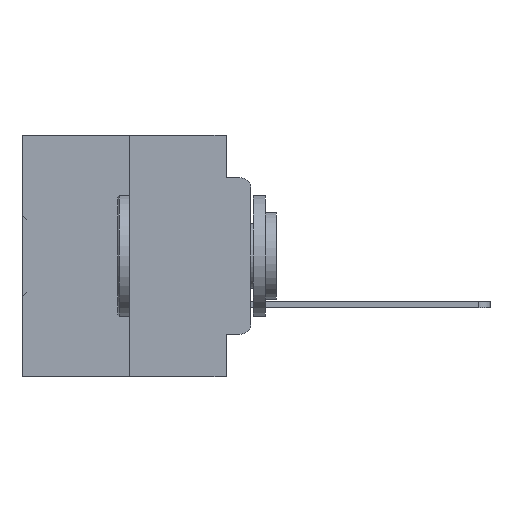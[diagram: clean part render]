
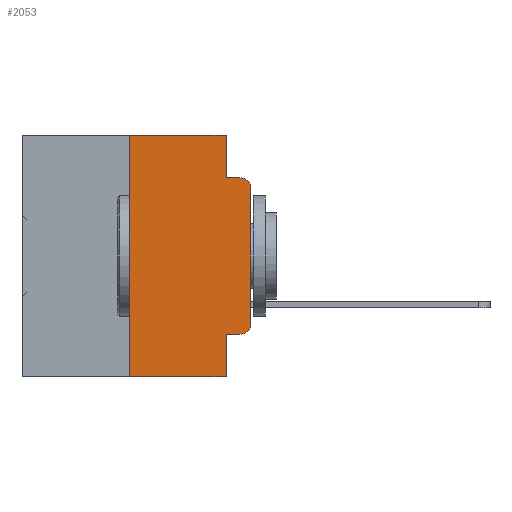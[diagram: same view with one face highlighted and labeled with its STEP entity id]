
A CAD part, left-side view. The second image highlights one B-rep face of the part: STEP entity #2053.
In plain terms, the highlighted planar face has unit normal (-1, 0, 0).
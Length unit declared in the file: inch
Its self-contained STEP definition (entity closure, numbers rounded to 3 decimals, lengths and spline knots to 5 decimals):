
#136 = EDGE_CURVE ( 'NONE', #15803, #18637, #18666, .T. ) ;
#483 = VECTOR ( 'NONE', #5728, 39.37008 ) ;
#659 = CARTESIAN_POINT ( 'NONE',  ( 0., 0.051, 0. ) ) ;
#1601 = VECTOR ( 'NONE', #25866, 39.37008 ) ;
#1630 = DIRECTION ( 'NONE',  ( 0., 0., -1. ) ) ;
#2053 = ADVANCED_FACE ( 'NONE', ( #24489 ), #9906, .F. ) ;
#2297 = ORIENTED_EDGE ( 'NONE', *, *, #10276, .F. ) ;
#2713 = CARTESIAN_POINT ( 'NONE',  ( 0., 0., 0. ) ) ;
#2790 = CARTESIAN_POINT ( 'NONE',  ( 0., 0., -0.1085 ) ) ;
#3482 = EDGE_CURVE ( 'NONE', #35715, #7925, #32908, .T. ) ;
#3700 = VERTEX_POINT ( 'NONE', #659 ) ;
#3823 = ORIENTED_EDGE ( 'NONE', *, *, #28074, .T. ) ;
#4172 = VERTEX_POINT ( 'NONE', #6162 ) ;
#4455 = LINE ( 'NONE', #8691, #10554 ) ;
#4606 = VERTEX_POINT ( 'NONE', #23449 ) ;
#4635 = LINE ( 'NONE', #26584, #33056 ) ;
#5728 = DIRECTION ( 'NONE',  ( 0., -1., 0. ) ) ;
#5882 = CARTESIAN_POINT ( 'NONE',  ( 0., 0.051, -0.5 ) ) ;
#6162 = CARTESIAN_POINT ( 'NONE',  ( 0., 0.051, -0.0885 ) ) ;
#6671 = CIRCLE ( 'NONE', #35570, 0.02 ) ;
#7572 = ORIENTED_EDGE ( 'NONE', *, *, #29208, .F. ) ;
#7925 = VERTEX_POINT ( 'NONE', #2790 ) ;
#8540 = CARTESIAN_POINT ( 'NONE',  ( 0., 0.051, 0. ) ) ;
#8691 = CARTESIAN_POINT ( 'NONE',  ( 0., 0.051, 0. ) ) ;
#9240 = DIRECTION ( 'NONE',  ( 0., 0., -1. ) ) ;
#9470 = DIRECTION ( 'NONE',  ( 0., -1., 0. ) ) ;
#9844 = CARTESIAN_POINT ( 'NONE',  ( 0., 0.051, -0.4115 ) ) ;
#9847 = DIRECTION ( 'NONE',  ( 1., 0., 0. ) ) ;
#9906 = PLANE ( 'NONE',  #11166 ) ;
#10276 = EDGE_CURVE ( 'NONE', #4606, #31587, #27240, .T. ) ;
#10360 = DIRECTION ( 'NONE',  ( 0., 0., -1. ) ) ;
#10416 = LINE ( 'NONE', #11674, #483 ) ;
#10554 = VECTOR ( 'NONE', #28633, 39.37008 ) ;
#11166 = AXIS2_PLACEMENT_3D ( 'NONE', #29204, #9847, #10360 ) ;
#11674 = CARTESIAN_POINT ( 'NONE',  ( 0., 0.051, -0.0885 ) ) ;
#11738 = VECTOR ( 'NONE', #9470, 39.37008 ) ;
#14117 = EDGE_LOOP ( 'NONE', ( #24926, #21089, #7572, #34600, #26935, #2297, #33570, #34814, #3823, #26265 ) ) ;
#15803 = VERTEX_POINT ( 'NONE', #35841 ) ;
#16489 = CIRCLE ( 'NONE', #26472, 0.02 ) ;
#16512 = DIRECTION ( 'NONE',  ( -1., 0., 0. ) ) ;
#17575 = CARTESIAN_POINT ( 'NONE',  ( 0., 0.25, 0. ) ) ;
#17732 = VERTEX_POINT ( 'NONE', #24261 ) ;
#18200 = VECTOR ( 'NONE', #22264, 39.37008 ) ;
#18544 = CARTESIAN_POINT ( 'NONE',  ( 0., 0.02, -0.4115 ) ) ;
#18637 = VERTEX_POINT ( 'NONE', #5882 ) ;
#18666 = LINE ( 'NONE', #8540, #32355 ) ;
#19389 = DIRECTION ( 'NONE',  ( -1., 0., 0. ) ) ;
#21068 = DIRECTION ( 'NONE',  ( 0., -1., 0. ) ) ;
#21089 = ORIENTED_EDGE ( 'NONE', *, *, #32834, .T. ) ;
#21883 = EDGE_CURVE ( 'NONE', #3700, #4172, #4455, .T. ) ;
#22264 = DIRECTION ( 'NONE',  ( 0., 0., 1. ) ) ;
#22283 = LINE ( 'NONE', #9844, #28720 ) ;
#23449 = CARTESIAN_POINT ( 'NONE',  ( 0., 0.25, -0.5 ) ) ;
#23805 = CARTESIAN_POINT ( 'NONE',  ( 0., 0.473, 0. ) ) ;
#24261 = CARTESIAN_POINT ( 'NONE',  ( 0., 0.02, -0.0885 ) ) ;
#24369 = EDGE_CURVE ( 'NONE', #29424, #35715, #6671, .T. ) ;
#24489 = FACE_OUTER_BOUND ( 'NONE', #14117, .T. ) ;
#24926 = ORIENTED_EDGE ( 'NONE', *, *, #3482, .T. ) ;
#25866 = DIRECTION ( 'NONE',  ( 0., 0., 1. ) ) ;
#26265 = ORIENTED_EDGE ( 'NONE', *, *, #24369, .T. ) ;
#26468 = CARTESIAN_POINT ( 'NONE',  ( 0., 0., -0.3915 ) ) ;
#26472 = AXIS2_PLACEMENT_3D ( 'NONE', #32925, #16512, #35614 ) ;
#26584 = CARTESIAN_POINT ( 'NONE',  ( 0., 0.473, -0.5 ) ) ;
#26906 = DIRECTION ( 'NONE',  ( 0., -1., 0. ) ) ;
#26935 = ORIENTED_EDGE ( 'NONE', *, *, #34165, .F. ) ;
#27240 = LINE ( 'NONE', #30405, #18200 ) ;
#28074 = EDGE_CURVE ( 'NONE', #15803, #29424, #22283, .T. ) ;
#28633 = DIRECTION ( 'NONE',  ( 0., 0., -1. ) ) ;
#28720 = VECTOR ( 'NONE', #26906, 39.37008 ) ;
#29204 = CARTESIAN_POINT ( 'NONE',  ( 0., 0.473, 0. ) ) ;
#29208 = EDGE_CURVE ( 'NONE', #4172, #17732, #10416, .T. ) ;
#29424 = VERTEX_POINT ( 'NONE', #18544 ) ;
#30405 = CARTESIAN_POINT ( 'NONE',  ( 0., 0.25, 0. ) ) ;
#31587 = VERTEX_POINT ( 'NONE', #17575 ) ;
#31768 = EDGE_CURVE ( 'NONE', #4606, #18637, #4635, .T. ) ;
#32355 = VECTOR ( 'NONE', #9240, 39.37008 ) ;
#32834 = EDGE_CURVE ( 'NONE', #7925, #17732, #16489, .T. ) ;
#32908 = LINE ( 'NONE', #2713, #1601 ) ;
#32925 = CARTESIAN_POINT ( 'NONE',  ( 0., 0.02, -0.1085 ) ) ;
#33056 = VECTOR ( 'NONE', #21068, 39.37008 ) ;
#33097 = LINE ( 'NONE', #23805, #11738 ) ;
#33570 = ORIENTED_EDGE ( 'NONE', *, *, #31768, .T. ) ;
#34165 = EDGE_CURVE ( 'NONE', #31587, #3700, #33097, .T. ) ;
#34600 = ORIENTED_EDGE ( 'NONE', *, *, #21883, .F. ) ;
#34814 = ORIENTED_EDGE ( 'NONE', *, *, #136, .F. ) ;
#35570 = AXIS2_PLACEMENT_3D ( 'NONE', #35685, #19389, #1630 ) ;
#35614 = DIRECTION ( 'NONE',  ( 0., 0., -1. ) ) ;
#35685 = CARTESIAN_POINT ( 'NONE',  ( 0., 0.02, -0.3915 ) ) ;
#35715 = VERTEX_POINT ( 'NONE', #26468 ) ;
#35841 = CARTESIAN_POINT ( 'NONE',  ( 0., 0.051, -0.4115 ) ) ;
